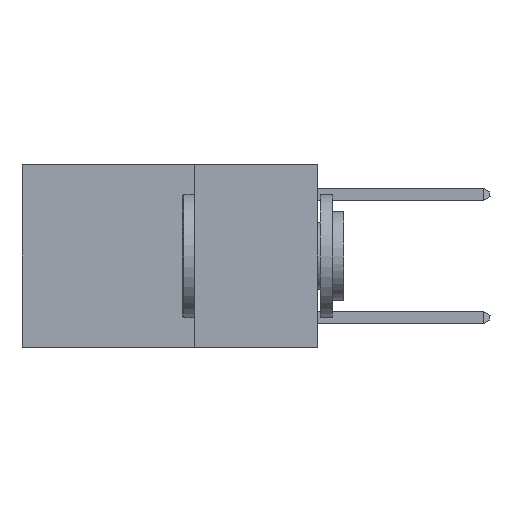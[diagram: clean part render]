
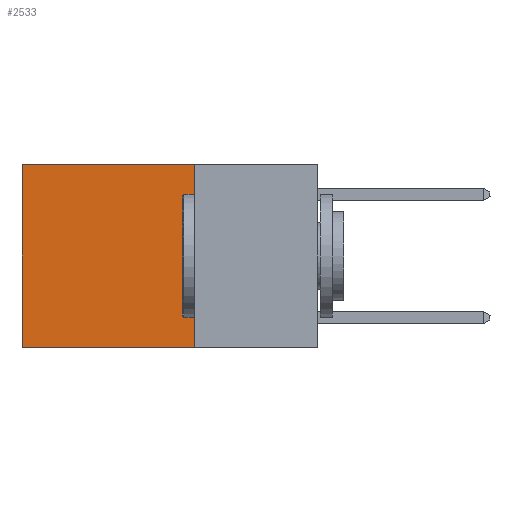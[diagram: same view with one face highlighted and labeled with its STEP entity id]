
A CAD part, left-side view. The second image highlights one B-rep face of the part: STEP entity #2533.
In plain terms, the highlighted planar face has unit normal (-1, 0, 0).
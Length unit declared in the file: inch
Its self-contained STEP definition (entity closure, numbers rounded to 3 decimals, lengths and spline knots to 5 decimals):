
#427 = VECTOR ( 'NONE', #8116, 39.37008 ) ;
#477 = DIRECTION ( 'NONE',  ( 1., 0., 0. ) ) ;
#933 = VERTEX_POINT ( 'NONE', #15299 ) ;
#2533 = ADVANCED_FACE ( 'NONE', ( #13631 ), #9733, .F. ) ;
#2765 = CARTESIAN_POINT ( 'NONE',  ( 0.2625, 0.25, 0. ) ) ;
#3278 = EDGE_CURVE ( 'NONE', #9827, #933, #7802, .T. ) ;
#3783 = CARTESIAN_POINT ( 'NONE',  ( 0.2625, 0.25, 0. ) ) ;
#4761 = VECTOR ( 'NONE', #4801, 39.37008 ) ;
#4801 = DIRECTION ( 'NONE',  ( 0., 1., 0. ) ) ;
#5763 = DIRECTION ( 'NONE',  ( 0., 0., -1. ) ) ;
#6121 = DIRECTION ( 'NONE',  ( 0., 1., 0. ) ) ;
#6324 = CARTESIAN_POINT ( 'NONE',  ( 0.2625, 0.6, 0. ) ) ;
#6355 = CARTESIAN_POINT ( 'NONE',  ( 0.2625, 0.25, -0.37 ) ) ;
#6509 = ORIENTED_EDGE ( 'NONE', *, *, #3278, .T. ) ;
#6821 = CARTESIAN_POINT ( 'NONE',  ( 0.2625, 0.25, 0. ) ) ;
#6903 = LINE ( 'NONE', #2765, #427 ) ;
#7058 = CARTESIAN_POINT ( 'NONE',  ( 0.2625, 0.25, 0. ) ) ;
#7802 = LINE ( 'NONE', #6324, #9502 ) ;
#8049 = VERTEX_POINT ( 'NONE', #8409 ) ;
#8116 = DIRECTION ( 'NONE',  ( 0., 0., -1. ) ) ;
#8409 = CARTESIAN_POINT ( 'NONE',  ( 0.2625, 0.25, -0.37 ) ) ;
#8915 = VECTOR ( 'NONE', #6121, 39.37008 ) ;
#9109 = EDGE_CURVE ( 'NONE', #15932, #8049, #6903, .T. ) ;
#9502 = VECTOR ( 'NONE', #10395, 39.37008 ) ;
#9733 = PLANE ( 'NONE',  #16910 ) ;
#9815 = CARTESIAN_POINT ( 'NONE',  ( 0.2625, 0.6, 0. ) ) ;
#9823 = EDGE_LOOP ( 'NONE', ( #6509, #12745, #14035, #15316 ) ) ;
#9827 = VERTEX_POINT ( 'NONE', #9815 ) ;
#10250 = LINE ( 'NONE', #6355, #4761 ) ;
#10395 = DIRECTION ( 'NONE',  ( 0., 0., -1. ) ) ;
#12693 = LINE ( 'NONE', #3783, #8915 ) ;
#12745 = ORIENTED_EDGE ( 'NONE', *, *, #16590, .F. ) ;
#13631 = FACE_OUTER_BOUND ( 'NONE', #9823, .T. ) ;
#14035 = ORIENTED_EDGE ( 'NONE', *, *, #9109, .F. ) ;
#14857 = EDGE_CURVE ( 'NONE', #15932, #9827, #12693, .T. ) ;
#15299 = CARTESIAN_POINT ( 'NONE',  ( 0.2625, 0.6, -0.37 ) ) ;
#15316 = ORIENTED_EDGE ( 'NONE', *, *, #14857, .T. ) ;
#15932 = VERTEX_POINT ( 'NONE', #6821 ) ;
#16590 = EDGE_CURVE ( 'NONE', #8049, #933, #10250, .T. ) ;
#16910 = AXIS2_PLACEMENT_3D ( 'NONE', #7058, #477, #5763 ) ;
